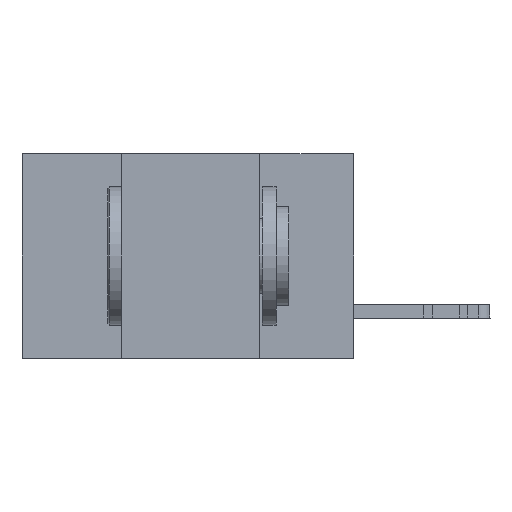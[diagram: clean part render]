
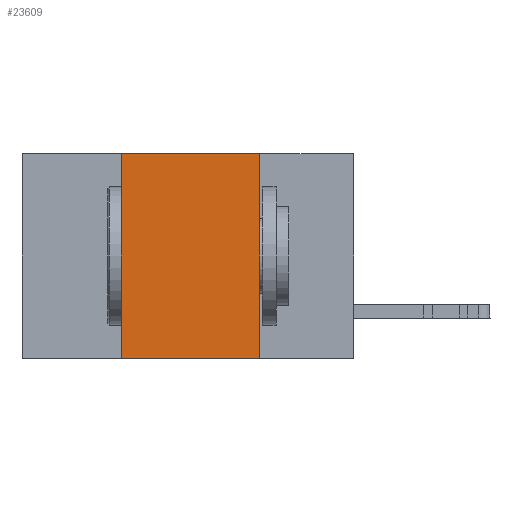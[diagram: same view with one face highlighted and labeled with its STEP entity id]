
A CAD part, left-side view. The second image highlights one B-rep face of the part: STEP entity #23609.
In plain terms, the highlighted planar face has unit normal (-1, 0, 0).
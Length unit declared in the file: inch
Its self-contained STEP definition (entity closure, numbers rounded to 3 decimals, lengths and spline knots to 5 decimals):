
#2224 = ORIENTED_EDGE ( 'NONE', *, *, #5475, .F. ) ;
#3570 = CARTESIAN_POINT ( 'NONE',  ( 0., 0.6, -0.37 ) ) ;
#3891 = CARTESIAN_POINT ( 'NONE',  ( 0., 0.42, 0. ) ) ;
#4554 = ORIENTED_EDGE ( 'NONE', *, *, #10928, .T. ) ;
#5475 = EDGE_CURVE ( 'NONE', #11757, #37278, #18032, .T. ) ;
#5665 = LINE ( 'NONE', #3570, #19180 ) ;
#7076 = CARTESIAN_POINT ( 'NONE',  ( 0., 0.17, -0.37 ) ) ;
#8335 = VERTEX_POINT ( 'NONE', #7076 ) ;
#10169 = ORIENTED_EDGE ( 'NONE', *, *, #13713, .F. ) ;
#10343 = FACE_OUTER_BOUND ( 'NONE', #26279, .T. ) ;
#10928 = EDGE_CURVE ( 'NONE', #32977, #8335, #5665, .T. ) ;
#11757 = VERTEX_POINT ( 'NONE', #40057 ) ;
#11978 = CARTESIAN_POINT ( 'NONE',  ( 0., 0.42, -0.37 ) ) ;
#13713 = EDGE_CURVE ( 'NONE', #37278, #8335, #29725, .T. ) ;
#17212 = AXIS2_PLACEMENT_3D ( 'NONE', #29986, #37092, #40543 ) ;
#18032 = LINE ( 'NONE', #26153, #19739 ) ;
#19180 = VECTOR ( 'NONE', #43539, 39.37008 ) ;
#19739 = VECTOR ( 'NONE', #20110, 39.37008 ) ;
#20110 = DIRECTION ( 'NONE',  ( 0., -1., 0. ) ) ;
#22423 = ORIENTED_EDGE ( 'NONE', *, *, #36931, .F. ) ;
#22577 = LINE ( 'NONE', #3891, #34503 ) ;
#23609 = ADVANCED_FACE ( 'NONE', ( #10343 ), #29359, .F. ) ;
#26153 = CARTESIAN_POINT ( 'NONE',  ( 0., 0.6, 0. ) ) ;
#26279 = EDGE_LOOP ( 'NONE', ( #10169, #2224, #22423, #4554 ) ) ;
#29359 = PLANE ( 'NONE',  #17212 ) ;
#29725 = LINE ( 'NONE', #42704, #35131 ) ;
#29986 = CARTESIAN_POINT ( 'NONE',  ( 0., 0.6, 0. ) ) ;
#31558 = DIRECTION ( 'NONE',  ( 0., 0., 1. ) ) ;
#32962 = DIRECTION ( 'NONE',  ( 0., 0., -1. ) ) ;
#32977 = VERTEX_POINT ( 'NONE', #11978 ) ;
#34020 = CARTESIAN_POINT ( 'NONE',  ( 0., 0.17, 0. ) ) ;
#34503 = VECTOR ( 'NONE', #31558, 39.37008 ) ;
#35131 = VECTOR ( 'NONE', #32962, 39.37008 ) ;
#36931 = EDGE_CURVE ( 'NONE', #32977, #11757, #22577, .T. ) ;
#37092 = DIRECTION ( 'NONE',  ( 1., 0., 0. ) ) ;
#37278 = VERTEX_POINT ( 'NONE', #34020 ) ;
#40057 = CARTESIAN_POINT ( 'NONE',  ( 0., 0.42, 0. ) ) ;
#40543 = DIRECTION ( 'NONE',  ( 0., 0., -1. ) ) ;
#42704 = CARTESIAN_POINT ( 'NONE',  ( 0., 0.17, 0. ) ) ;
#43539 = DIRECTION ( 'NONE',  ( 0., -1., 0. ) ) ;
